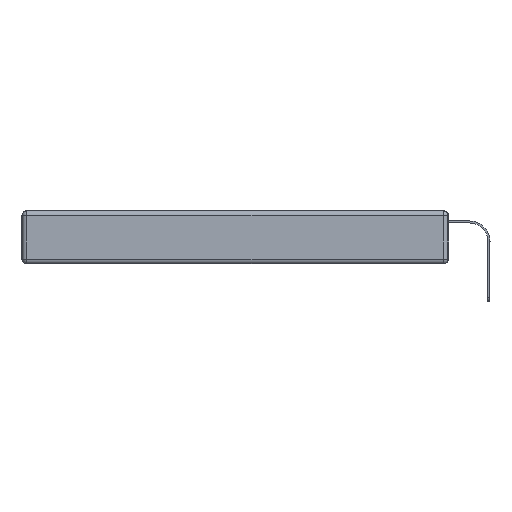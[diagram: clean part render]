
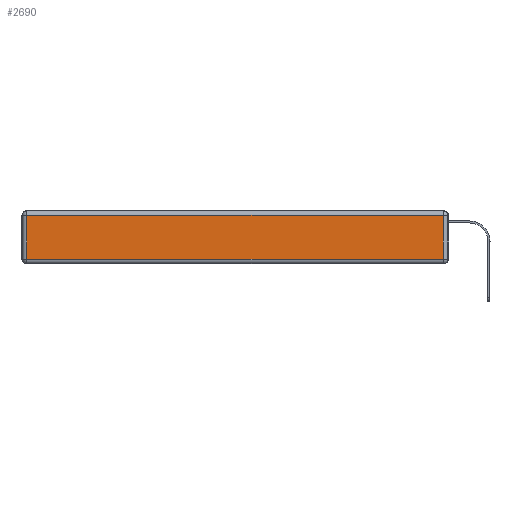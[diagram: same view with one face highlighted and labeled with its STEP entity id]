
A CAD part, left-side view. The second image highlights one B-rep face of the part: STEP entity #2690.
In plain terms, the highlighted planar face has unit normal (-1, 0, 0).
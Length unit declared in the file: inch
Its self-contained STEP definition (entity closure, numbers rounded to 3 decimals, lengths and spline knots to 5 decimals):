
#755 = CARTESIAN_POINT ( 'NONE',  ( 0., 0., -0.343 ) ) ;
#1585 = VERTEX_POINT ( 'NONE', #14783 ) ;
#2263 = EDGE_CURVE ( 'NONE', #7030, #18666, #16810, .T. ) ;
#2690 = ADVANCED_FACE ( 'NONE', ( #2890 ), #16334, .T. ) ;
#2890 = FACE_OUTER_BOUND ( 'NONE', #4529, .T. ) ;
#3102 = DIRECTION ( 'NONE',  ( 0., -1., 0. ) ) ;
#3743 = EDGE_CURVE ( 'NONE', #15151, #7030, #10577, .T. ) ;
#4477 = CARTESIAN_POINT ( 'NONE',  ( 0., 2.72, -0.313 ) ) ;
#4529 = EDGE_LOOP ( 'NONE', ( #14058, #11453, #6925, #17369 ) ) ;
#5057 = CARTESIAN_POINT ( 'NONE',  ( 0., 0.03, -0.343 ) ) ;
#6903 = VECTOR ( 'NONE', #15599, 39.37008 ) ;
#6925 = ORIENTED_EDGE ( 'NONE', *, *, #3743, .T. ) ;
#7030 = VERTEX_POINT ( 'NONE', #20366 ) ;
#7242 = AXIS2_PLACEMENT_3D ( 'NONE', #755, #7541, #7881 ) ;
#7541 = DIRECTION ( 'NONE',  ( -1., 0., 0. ) ) ;
#7843 = EDGE_CURVE ( 'NONE', #1585, #15151, #16840, .T. ) ;
#7881 = DIRECTION ( 'NONE',  ( 0., 0., 1. ) ) ;
#8646 = VECTOR ( 'NONE', #19728, 39.37008 ) ;
#10577 = LINE ( 'NONE', #20705, #6903 ) ;
#10637 = CARTESIAN_POINT ( 'NONE',  ( 0., 0.03, -0.03 ) ) ;
#11281 = EDGE_CURVE ( 'NONE', #18666, #1585, #21542, .T. ) ;
#11453 = ORIENTED_EDGE ( 'NONE', *, *, #7843, .T. ) ;
#11527 = CARTESIAN_POINT ( 'NONE',  ( 0., 0., -0.313 ) ) ;
#14058 = ORIENTED_EDGE ( 'NONE', *, *, #11281, .T. ) ;
#14783 = CARTESIAN_POINT ( 'NONE',  ( 0., 0.03, -0.313 ) ) ;
#15151 = VERTEX_POINT ( 'NONE', #10637 ) ;
#15599 = DIRECTION ( 'NONE',  ( 0., 1., 0. ) ) ;
#16334 = PLANE ( 'NONE',  #7242 ) ;
#16810 = LINE ( 'NONE', #18145, #8646 ) ;
#16840 = LINE ( 'NONE', #5057, #18307 ) ;
#17369 = ORIENTED_EDGE ( 'NONE', *, *, #2263, .T. ) ;
#18145 = CARTESIAN_POINT ( 'NONE',  ( 0., 2.72, -0.343 ) ) ;
#18307 = VECTOR ( 'NONE', #18726, 39.37008 ) ;
#18666 = VERTEX_POINT ( 'NONE', #4477 ) ;
#18726 = DIRECTION ( 'NONE',  ( 0., 0., 1. ) ) ;
#19728 = DIRECTION ( 'NONE',  ( 0., 0., -1. ) ) ;
#20366 = CARTESIAN_POINT ( 'NONE',  ( 0., 2.72, -0.03 ) ) ;
#20705 = CARTESIAN_POINT ( 'NONE',  ( 0., 2.75, -0.03 ) ) ;
#21277 = VECTOR ( 'NONE', #3102, 39.37008 ) ;
#21542 = LINE ( 'NONE', #11527, #21277 ) ;
